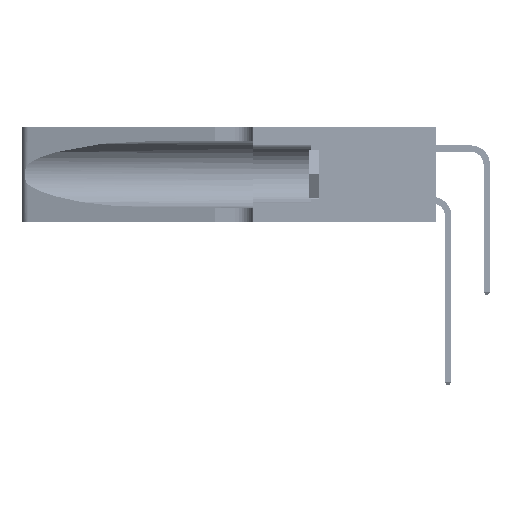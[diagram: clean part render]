
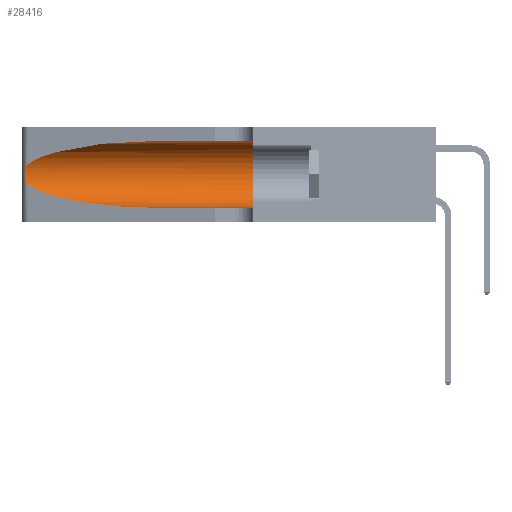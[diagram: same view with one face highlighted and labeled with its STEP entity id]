
A CAD part, left-side view. The second image highlights one B-rep face of the part: STEP entity #28416.
In plain terms, the highlighted cylindrical face has radius 3.308 mm (diameter 6.617 mm), a partial arc.
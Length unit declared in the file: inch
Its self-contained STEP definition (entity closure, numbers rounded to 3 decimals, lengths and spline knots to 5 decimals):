
#86 = ORIENTED_EDGE ( 'NONE', *, *, #47622, .F. ) ;
#727 = CARTESIAN_POINT ( 'NONE',  ( 0.1305, 1.61858, 0.185 ) ) ;
#900 = DIRECTION ( 'NONE',  ( 0., 0., -1. ) ) ;
#1732 = ORIENTED_EDGE ( 'NONE', *, *, #4960, .F. ) ;
#3689 = CIRCLE ( 'NONE', #15376, 0.13025 ) ;
#4371 = CARTESIAN_POINT ( 'NONE',  ( 0.25487, 1.22718, 0.14631 ) ) ;
#4960 = EDGE_CURVE ( 'NONE', #34892, #54134, #28408, .T. ) ;
#5181 = EDGE_CURVE ( 'NONE', #14130, #39527, #17882, .T. ) ;
#6033 = VECTOR ( 'NONE', #8750, 39.37008 ) ;
#6098 = CARTESIAN_POINT ( 'NONE',  ( 0.25787, 1.23484, 0.2124 ) ) ;
#8750 = DIRECTION ( 'NONE',  ( 0., -1., 0. ) ) ;
#8848 = ORIENTED_EDGE ( 'NONE', *, *, #33893, .T. ) ;
#10305 = CARTESIAN_POINT ( 'NONE',  ( 0.26018, 1.23835, 0.19895 ) ) ;
#12161 = CARTESIAN_POINT ( 'NONE',  ( 0.18966, 0.96281, 0.05475 ) ) ;
#13781 = ORIENTED_EDGE ( 'NONE', *, *, #19702, .T. ) ;
#14130 = VERTEX_POINT ( 'NONE', #52170 ) ;
#14559 = CARTESIAN_POINT ( 'NONE',  ( 0.26075, 1.23896, 0.178 ) ) ;
#14682 = EDGE_LOOP ( 'NONE', ( #8848, #19277, #13781, #46031, #86, #1732 ) ) ;
#15376 = AXIS2_PLACEMENT_3D ( 'NONE', #20301, #49724, #24502 ) ;
#15603 =( BOUNDED_CURVE ( )  B_SPLINE_CURVE ( 3, ( #32439, #15889, #49524, #24304 ),
 .UNSPECIFIED., .F., .T. ) 
 B_SPLINE_CURVE_WITH_KNOTS ( ( 4, 4 ),
 ( 1.5708, 2.84003 ),
 .UNSPECIFIED. ) 
 CURVE ( )  GEOMETRIC_REPRESENTATION_ITEM ( )  RATIONAL_B_SPLINE_CURVE ( ( 1., 0.87, 0.87, 1. ) ) 
 REPRESENTATION_ITEM ( '' )  );
#15889 = CARTESIAN_POINT ( 'NONE',  ( 0.18966, 0.96281, 0.31525 ) ) ;
#17240 = CARTESIAN_POINT ( 'NONE',  ( 0.1305, 1.61858, 0.31525 ) ) ;
#17882 = LINE ( 'NONE', #44606, #29063 ) ;
#18148 = CARTESIAN_POINT ( 'NONE',  ( 0.25487, 1.22718, 0.22369 ) ) ;
#18604 = CARTESIAN_POINT ( 'NONE',  ( 0.25487, 1.22718, 0.22369 ) ) ;
#18780 = CARTESIAN_POINT ( 'NONE',  ( 0.25856, 1.23593, 0.16098 ) ) ;
#19277 = ORIENTED_EDGE ( 'NONE', *, *, #30758, .T. ) ;
#19702 = EDGE_CURVE ( 'NONE', #22752, #14130, #41412, .T. ) ;
#20085 = CARTESIAN_POINT ( 'NONE',  ( 0.1305, 0.35, 0.05475 ) ) ;
#20301 = CARTESIAN_POINT ( 'NONE',  ( 0.1305, 0.35, 0.185 ) ) ;
#22752 = VERTEX_POINT ( 'NONE', #4371 ) ;
#22819 = CARTESIAN_POINT ( 'NONE',  ( 0.25555, 1.22994, 0.2215 ) ) ;
#22999 = CARTESIAN_POINT ( 'NONE',  ( 0.25639, 1.23186, 0.15144 ) ) ;
#24304 = CARTESIAN_POINT ( 'NONE',  ( 0.25487, 1.22718, 0.22369 ) ) ;
#24502 = DIRECTION ( 'NONE',  ( 0., 0., 1. ) ) ;
#27206 = CARTESIAN_POINT ( 'NONE',  ( 0.25487, 1.22718, 0.14631 ) ) ;
#28408 = LINE ( 'NONE', #17240, #6033 ) ;
#28416 = ADVANCED_FACE ( 'NONE', ( #39978 ), #28799, .F. ) ;
#28799 = CYLINDRICAL_SURFACE ( 'NONE', #32474, 0.13025 ) ;
#28890 = CARTESIAN_POINT ( 'NONE',  ( 0.25487, 1.22718, 0.14631 ) ) ;
#29063 = VECTOR ( 'NONE', #36117, 39.37008 ) ;
#30312 = CARTESIAN_POINT ( 'NONE',  ( 0.1305, 0.72297, 0.31525 ) ) ;
#30758 = EDGE_CURVE ( 'NONE', #51571, #22752, #37854, .T. ) ;
#31278 = CARTESIAN_POINT ( 'NONE',  ( 0.25639, 1.23184, 0.21858 ) ) ;
#32439 = CARTESIAN_POINT ( 'NONE',  ( 0.1305, 0.72297, 0.31525 ) ) ;
#32474 = AXIS2_PLACEMENT_3D ( 'NONE', #727, #51308, #900 ) ;
#33893 = EDGE_CURVE ( 'NONE', #34892, #51571, #15603, .T. ) ;
#34892 = VERTEX_POINT ( 'NONE', #30312 ) ;
#35526 = CARTESIAN_POINT ( 'NONE',  ( 0.25854, 1.2359, 0.20912 ) ) ;
#36117 = DIRECTION ( 'NONE',  ( 0., -1., 0. ) ) ;
#37854 = B_SPLINE_CURVE_WITH_KNOTS ( 'NONE', 3,
 ( #18604, #22819, #31278, #6098, #35526, #10305, #39743, #14559, #43995, #18780, #48192, #22999, #52465, #27206 ),
 .UNSPECIFIED., .F., .F.,
 ( 4, 2, 2, 2, 2, 2, 4 ),
 ( 0., 0.00027, 0.00053, 0.00107, 0.0016, 0.00187, 0.00214 ),
 .UNSPECIFIED. ) ;
#39527 = VERTEX_POINT ( 'NONE', #20085 ) ;
#39743 = CARTESIAN_POINT ( 'NONE',  ( 0.26075, 1.23896, 0.19203 ) ) ;
#39978 = FACE_OUTER_BOUND ( 'NONE', #14682, .T. ) ;
#41412 =( BOUNDED_CURVE ( )  B_SPLINE_CURVE ( 3, ( #28890, #54108, #12161, #41603 ),
 .UNSPECIFIED., .F., .T. ) 
 B_SPLINE_CURVE_WITH_KNOTS ( ( 4, 4 ),
 ( 3.44316, 4.71239 ),
 .UNSPECIFIED. ) 
 CURVE ( )  GEOMETRIC_REPRESENTATION_ITEM ( )  RATIONAL_B_SPLINE_CURVE ( ( 1., 0.87, 0.87, 1. ) ) 
 REPRESENTATION_ITEM ( '' )  );
#41603 = CARTESIAN_POINT ( 'NONE',  ( 0.1305, 0.72297, 0.05475 ) ) ;
#43995 = CARTESIAN_POINT ( 'NONE',  ( 0.26017, 1.23833, 0.17102 ) ) ;
#44606 = CARTESIAN_POINT ( 'NONE',  ( 0.1305, 1.61858, 0.05475 ) ) ;
#46031 = ORIENTED_EDGE ( 'NONE', *, *, #5181, .T. ) ;
#47622 = EDGE_CURVE ( 'NONE', #54134, #39527, #3689, .T. ) ;
#48192 = CARTESIAN_POINT ( 'NONE',  ( 0.25789, 1.23486, 0.15765 ) ) ;
#48433 = CARTESIAN_POINT ( 'NONE',  ( 0.1305, 0.35, 0.31525 ) ) ;
#49524 = CARTESIAN_POINT ( 'NONE',  ( 0.2373, 1.15595, 0.28018 ) ) ;
#49724 = DIRECTION ( 'NONE',  ( 0., 1., 0. ) ) ;
#51308 = DIRECTION ( 'NONE',  ( 0., -1., 0. ) ) ;
#51571 = VERTEX_POINT ( 'NONE', #18148 ) ;
#52170 = CARTESIAN_POINT ( 'NONE',  ( 0.1305, 0.72297, 0.05475 ) ) ;
#52465 = CARTESIAN_POINT ( 'NONE',  ( 0.25555, 1.22993, 0.14849 ) ) ;
#54108 = CARTESIAN_POINT ( 'NONE',  ( 0.2373, 1.15595, 0.08982 ) ) ;
#54134 = VERTEX_POINT ( 'NONE', #48433 ) ;
